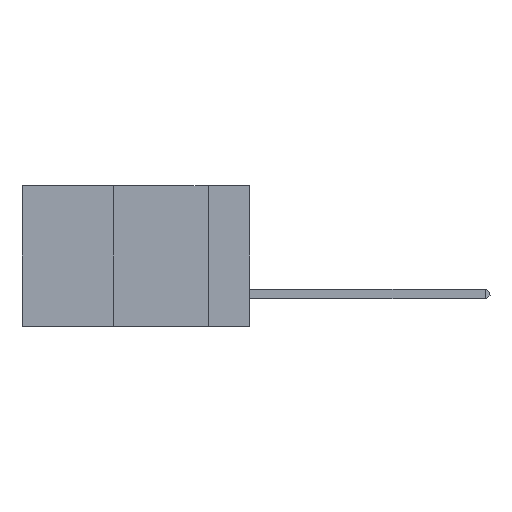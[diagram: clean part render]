
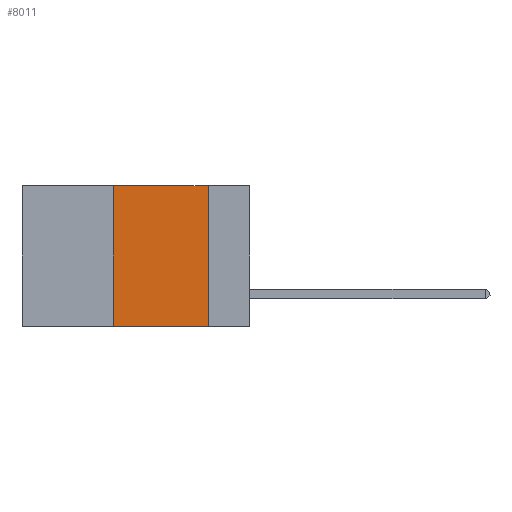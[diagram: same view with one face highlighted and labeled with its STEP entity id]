
A CAD part, left-side view. The second image highlights one B-rep face of the part: STEP entity #8011.
In plain terms, the highlighted planar face has unit normal (-1, 0, 0).
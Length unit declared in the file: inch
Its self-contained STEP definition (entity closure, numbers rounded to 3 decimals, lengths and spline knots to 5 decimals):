
#151 = EDGE_LOOP ( 'NONE', ( #8579, #982, #1044, #7488 ) ) ;
#709 = VERTEX_POINT ( 'NONE', #13026 ) ;
#875 = CARTESIAN_POINT ( 'NONE',  ( 0., 0.11, -0.37 ) ) ;
#982 = ORIENTED_EDGE ( 'NONE', *, *, #7861, .F. ) ;
#983 = AXIS2_PLACEMENT_3D ( 'NONE', #12431, #3995, #11042 ) ;
#1044 = ORIENTED_EDGE ( 'NONE', *, *, #11354, .F. ) ;
#1286 = LINE ( 'NONE', #10653, #9726 ) ;
#1858 = EDGE_CURVE ( 'NONE', #14175, #9760, #4202, .T. ) ;
#3798 = VECTOR ( 'NONE', #8112, 39.37008 ) ;
#3802 = PLANE ( 'NONE',  #983 ) ;
#3995 = DIRECTION ( 'NONE',  ( 1., 0., 0. ) ) ;
#4174 = LINE ( 'NONE', #15423, #3798 ) ;
#4202 = LINE ( 'NONE', #13507, #11396 ) ;
#4667 = FACE_OUTER_BOUND ( 'NONE', #151, .T. ) ;
#6029 = DIRECTION ( 'NONE',  ( 0., -1., 0. ) ) ;
#6145 = DIRECTION ( 'NONE',  ( 0., -1., 0. ) ) ;
#6148 = DIRECTION ( 'NONE',  ( 0., 0., -1. ) ) ;
#7411 = CARTESIAN_POINT ( 'NONE',  ( 0., 0.6, -0.37 ) ) ;
#7488 = ORIENTED_EDGE ( 'NONE', *, *, #12281, .T. ) ;
#7861 = EDGE_CURVE ( 'NONE', #709, #14175, #1286, .T. ) ;
#8011 = ADVANCED_FACE ( 'NONE', ( #4667 ), #3802, .F. ) ;
#8112 = DIRECTION ( 'NONE',  ( 0., 0., 1. ) ) ;
#8579 = ORIENTED_EDGE ( 'NONE', *, *, #1858, .F. ) ;
#9726 = VECTOR ( 'NONE', #6029, 39.37008 ) ;
#9760 = VERTEX_POINT ( 'NONE', #875 ) ;
#10118 = VECTOR ( 'NONE', #6145, 39.37008 ) ;
#10588 = CARTESIAN_POINT ( 'NONE',  ( 0., 0.11, 0. ) ) ;
#10653 = CARTESIAN_POINT ( 'NONE',  ( 0., 0.6, 0. ) ) ;
#11042 = DIRECTION ( 'NONE',  ( 0., 0., -1. ) ) ;
#11354 = EDGE_CURVE ( 'NONE', #13358, #709, #4174, .T. ) ;
#11396 = VECTOR ( 'NONE', #6148, 39.37008 ) ;
#11466 = LINE ( 'NONE', #7411, #10118 ) ;
#12281 = EDGE_CURVE ( 'NONE', #13358, #9760, #11466, .T. ) ;
#12431 = CARTESIAN_POINT ( 'NONE',  ( 0., 0.6, 0. ) ) ;
#13026 = CARTESIAN_POINT ( 'NONE',  ( 0., 0.36, 0. ) ) ;
#13358 = VERTEX_POINT ( 'NONE', #13647 ) ;
#13507 = CARTESIAN_POINT ( 'NONE',  ( 0., 0.11, 0. ) ) ;
#13647 = CARTESIAN_POINT ( 'NONE',  ( 0., 0.36, -0.37 ) ) ;
#14175 = VERTEX_POINT ( 'NONE', #10588 ) ;
#15423 = CARTESIAN_POINT ( 'NONE',  ( 0., 0.36, 0. ) ) ;
